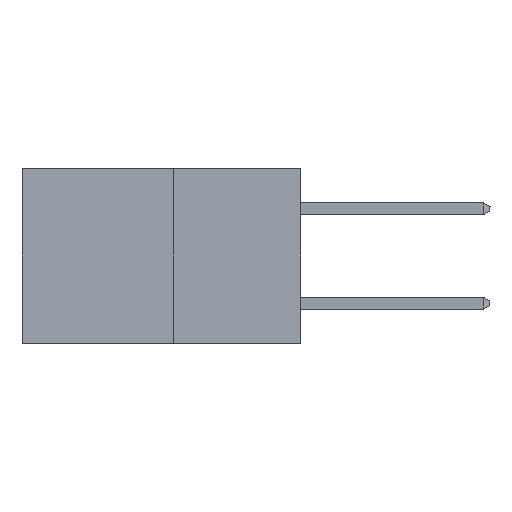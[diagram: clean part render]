
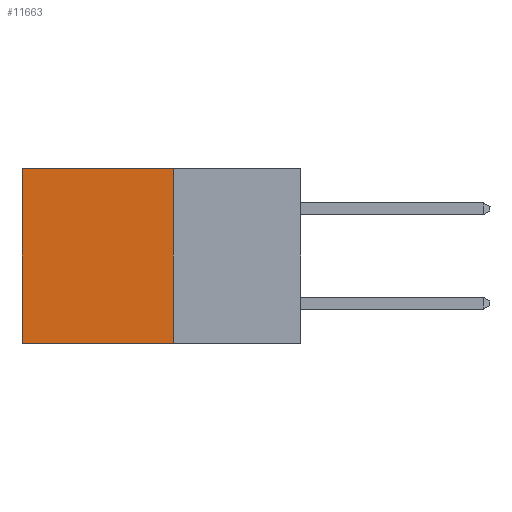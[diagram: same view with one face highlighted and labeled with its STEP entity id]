
A CAD part, left-side view. The second image highlights one B-rep face of the part: STEP entity #11663.
In plain terms, the highlighted planar face has unit normal (-1, 0, 0).
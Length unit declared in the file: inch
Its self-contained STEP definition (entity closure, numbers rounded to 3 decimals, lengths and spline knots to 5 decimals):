
#116 = ORIENTED_EDGE ( 'NONE', *, *, #3895, .T. ) ;
#345 = ORIENTED_EDGE ( 'NONE', *, *, #11081, .F. ) ;
#810 = LINE ( 'NONE', #15706, #15452 ) ;
#2117 = LINE ( 'NONE', #3465, #5386 ) ;
#2209 = AXIS2_PLACEMENT_3D ( 'NONE', #15297, #11262, #2886 ) ;
#2886 = DIRECTION ( 'NONE',  ( 0., 0., -1. ) ) ;
#3055 = CARTESIAN_POINT ( 'NONE',  ( 0.277, 0.59, -0.37 ) ) ;
#3073 = DIRECTION ( 'NONE',  ( 0., 1., 0. ) ) ;
#3465 = CARTESIAN_POINT ( 'NONE',  ( 0.277, 0.27, -0.37 ) ) ;
#3468 = DIRECTION ( 'NONE',  ( 0., 0., -1. ) ) ;
#3794 = EDGE_CURVE ( 'NONE', #10721, #14123, #6344, .T. ) ;
#3895 = EDGE_CURVE ( 'NONE', #14123, #17122, #810, .T. ) ;
#5386 = VECTOR ( 'NONE', #3468, 39.37008 ) ;
#5511 = EDGE_CURVE ( 'NONE', #17818, #17122, #8518, .T. ) ;
#5683 = CARTESIAN_POINT ( 'NONE',  ( 0.277, 0.27, -0.37 ) ) ;
#6344 = LINE ( 'NONE', #17983, #13484 ) ;
#6472 = CARTESIAN_POINT ( 'NONE',  ( 0.277, 0.27, 0. ) ) ;
#7120 = FACE_OUTER_BOUND ( 'NONE', #16927, .T. ) ;
#7592 = CARTESIAN_POINT ( 'NONE',  ( 0.277, 0.27, -0.37 ) ) ;
#8278 = ORIENTED_EDGE ( 'NONE', *, *, #3794, .T. ) ;
#8518 = LINE ( 'NONE', #5683, #12783 ) ;
#9300 = DIRECTION ( 'NONE',  ( 0., 1., 0. ) ) ;
#9847 = PLANE ( 'NONE',  #2209 ) ;
#10310 = ORIENTED_EDGE ( 'NONE', *, *, #5511, .F. ) ;
#10721 = VERTEX_POINT ( 'NONE', #6472 ) ;
#11081 = EDGE_CURVE ( 'NONE', #10721, #17818, #2117, .T. ) ;
#11262 = DIRECTION ( 'NONE',  ( 1., 0., 0. ) ) ;
#11663 = ADVANCED_FACE ( 'NONE', ( #7120 ), #9847, .F. ) ;
#12783 = VECTOR ( 'NONE', #3073, 39.37008 ) ;
#13484 = VECTOR ( 'NONE', #9300, 39.37008 ) ;
#14123 = VERTEX_POINT ( 'NONE', #17712 ) ;
#15297 = CARTESIAN_POINT ( 'NONE',  ( 0.277, 0.27, -0.37 ) ) ;
#15452 = VECTOR ( 'NONE', #17252, 39.37008 ) ;
#15706 = CARTESIAN_POINT ( 'NONE',  ( 0.277, 0.59, -0.37 ) ) ;
#16927 = EDGE_LOOP ( 'NONE', ( #116, #10310, #345, #8278 ) ) ;
#17122 = VERTEX_POINT ( 'NONE', #3055 ) ;
#17252 = DIRECTION ( 'NONE',  ( 0., 0., -1. ) ) ;
#17712 = CARTESIAN_POINT ( 'NONE',  ( 0.277, 0.59, 0. ) ) ;
#17818 = VERTEX_POINT ( 'NONE', #7592 ) ;
#17983 = CARTESIAN_POINT ( 'NONE',  ( 0.277, 0.27, 0. ) ) ;
